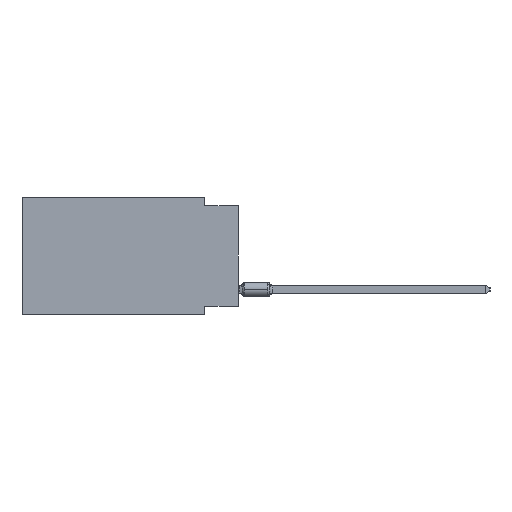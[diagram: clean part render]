
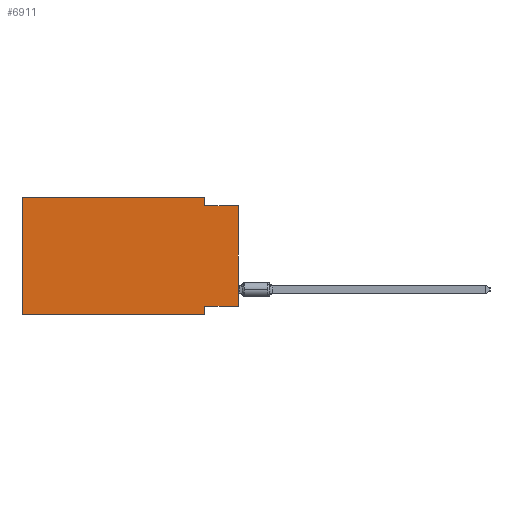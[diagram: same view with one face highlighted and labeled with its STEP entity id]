
A CAD part, left-side view. The second image highlights one B-rep face of the part: STEP entity #6911.
In plain terms, the highlighted planar face has unit normal (-1, 0, 0).
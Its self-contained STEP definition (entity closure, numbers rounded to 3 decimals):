
#747 = ORIENTED_EDGE ( 'NONE', *, *, #20975, .F. ) ;
#1677 = EDGE_CURVE ( 'NONE', #30695, #58925, #27542, .T. ) ;
#2005 = ORIENTED_EDGE ( 'NONE', *, *, #30435, .F. ) ;
#2055 = DIRECTION ( 'NONE',  ( 0., 0., -1. ) ) ;
#5175 = LINE ( 'NONE', #53540, #62926 ) ;
#6911 = ADVANCED_FACE ( 'NONE', ( #45602 ), #55511, .F. ) ;
#8216 = CARTESIAN_POINT ( 'NONE',  ( 0., 2.54, -0.635 ) ) ;
#8657 = CARTESIAN_POINT ( 'NONE',  ( 0., 16.383, -8.89 ) ) ;
#11610 = ORIENTED_EDGE ( 'NONE', *, *, #23807, .F. ) ;
#12056 = CARTESIAN_POINT ( 'NONE',  ( 0., 0., -8.255 ) ) ;
#12802 = VERTEX_POINT ( 'NONE', #15347 ) ;
#13084 = DIRECTION ( 'NONE',  ( 0., 0., 1. ) ) ;
#15347 = CARTESIAN_POINT ( 'NONE',  ( 0., 16.383, -8.89 ) ) ;
#15711 = CARTESIAN_POINT ( 'NONE',  ( 0., 0., -0.635 ) ) ;
#18391 = DIRECTION ( 'NONE',  ( 0., -1., 0. ) ) ;
#19076 = VERTEX_POINT ( 'NONE', #12056 ) ;
#19101 = EDGE_CURVE ( 'NONE', #58925, #58233, #22982, .T. ) ;
#19473 = EDGE_LOOP ( 'NONE', ( #22023, #38133, #50792, #39351, #2005, #44725, #11610, #747 ) ) ;
#20975 = EDGE_CURVE ( 'NONE', #19076, #62566, #50360, .T. ) ;
#22023 = ORIENTED_EDGE ( 'NONE', *, *, #47235, .T. ) ;
#22751 = DIRECTION ( 'NONE',  ( 0., 0., -1. ) ) ;
#22982 = LINE ( 'NONE', #46026, #54008 ) ;
#23399 = LINE ( 'NONE', #8657, #26908 ) ;
#23629 = VECTOR ( 'NONE', #18391, 1000. ) ;
#23684 = CARTESIAN_POINT ( 'NONE',  ( 0., 2.54, -8.89 ) ) ;
#23807 = EDGE_CURVE ( 'NONE', #62566, #51601, #5175, .T. ) ;
#25390 = DIRECTION ( 'NONE',  ( 0., 1., 0. ) ) ;
#26908 = VECTOR ( 'NONE', #28212, 1000. ) ;
#27071 = LINE ( 'NONE', #42103, #23629 ) ;
#27542 = LINE ( 'NONE', #47060, #55577 ) ;
#28212 = DIRECTION ( 'NONE',  ( 0., -1., 0. ) ) ;
#29318 = CARTESIAN_POINT ( 'NONE',  ( 0., 2.54, -8.255 ) ) ;
#30040 = CARTESIAN_POINT ( 'NONE',  ( 0., 2.54, 0. ) ) ;
#30435 = EDGE_CURVE ( 'NONE', #12802, #54292, #57579, .T. ) ;
#30695 = VERTEX_POINT ( 'NONE', #30040 ) ;
#32061 = DIRECTION ( 'NONE',  ( 0., 0., 1. ) ) ;
#33650 = VECTOR ( 'NONE', #32061, 1000. ) ;
#36739 = DIRECTION ( 'NONE',  ( 0., -1., 0. ) ) ;
#36865 = LINE ( 'NONE', #56379, #33650 ) ;
#38133 = ORIENTED_EDGE ( 'NONE', *, *, #19101, .F. ) ;
#39351 = ORIENTED_EDGE ( 'NONE', *, *, #45136, .F. ) ;
#40449 = CARTESIAN_POINT ( 'NONE',  ( 0., 0., -8.255 ) ) ;
#42103 = CARTESIAN_POINT ( 'NONE',  ( 0., 16.383, 0. ) ) ;
#43611 = DIRECTION ( 'NONE',  ( 0., 0., -1. ) ) ;
#44725 = ORIENTED_EDGE ( 'NONE', *, *, #55917, .T. ) ;
#45136 = EDGE_CURVE ( 'NONE', #54292, #30695, #27071, .T. ) ;
#45602 = FACE_OUTER_BOUND ( 'NONE', #19473, .T. ) ;
#45910 = CARTESIAN_POINT ( 'NONE',  ( 0., 16.383, 0. ) ) ;
#46026 = CARTESIAN_POINT ( 'NONE',  ( 0., 0., -0.635 ) ) ;
#47060 = CARTESIAN_POINT ( 'NONE',  ( 0., 2.54, 0. ) ) ;
#47235 = EDGE_CURVE ( 'NONE', #19076, #58233, #36865, .T. ) ;
#47857 = VECTOR ( 'NONE', #13084, 1000. ) ;
#50360 = LINE ( 'NONE', #40449, #52264 ) ;
#50401 = DIRECTION ( 'NONE',  ( 1., 0., 0. ) ) ;
#50792 = ORIENTED_EDGE ( 'NONE', *, *, #1677, .F. ) ;
#51601 = VERTEX_POINT ( 'NONE', #23684 ) ;
#52264 = VECTOR ( 'NONE', #25390, 1000. ) ;
#53540 = CARTESIAN_POINT ( 'NONE',  ( 0., 2.54, -8.89 ) ) ;
#54008 = VECTOR ( 'NONE', #36739, 1000. ) ;
#54292 = VERTEX_POINT ( 'NONE', #59691 ) ;
#55511 = PLANE ( 'NONE',  #63144 ) ;
#55577 = VECTOR ( 'NONE', #22751, 1000. ) ;
#55917 = EDGE_CURVE ( 'NONE', #12802, #51601, #23399, .T. ) ;
#56379 = CARTESIAN_POINT ( 'NONE',  ( 0., 0., 0. ) ) ;
#57579 = LINE ( 'NONE', #62708, #47857 ) ;
#58233 = VERTEX_POINT ( 'NONE', #15711 ) ;
#58925 = VERTEX_POINT ( 'NONE', #8216 ) ;
#59691 = CARTESIAN_POINT ( 'NONE',  ( 0., 16.383, 0. ) ) ;
#62566 = VERTEX_POINT ( 'NONE', #29318 ) ;
#62708 = CARTESIAN_POINT ( 'NONE',  ( 0., 16.383, 0. ) ) ;
#62926 = VECTOR ( 'NONE', #43611, 1000. ) ;
#63144 = AXIS2_PLACEMENT_3D ( 'NONE', #45910, #50401, #2055 ) ;
